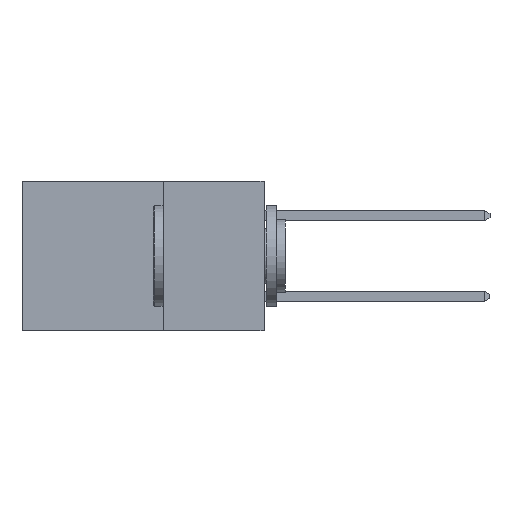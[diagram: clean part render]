
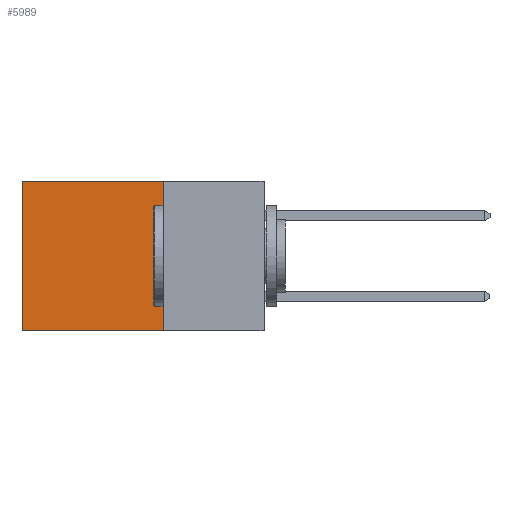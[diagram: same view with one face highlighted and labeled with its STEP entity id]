
A CAD part, left-side view. The second image highlights one B-rep face of the part: STEP entity #5989.
In plain terms, the highlighted planar face has unit normal (-1, 0, 0).
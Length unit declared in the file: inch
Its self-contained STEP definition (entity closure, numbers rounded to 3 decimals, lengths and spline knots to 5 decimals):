
#68 = LINE ( 'NONE', #2925, #7213 ) ;
#701 = ORIENTED_EDGE ( 'NONE', *, *, #2954, .F. ) ;
#1047 = CARTESIAN_POINT ( 'NONE',  ( 0.2615, 0.25, 0. ) ) ;
#1119 = ORIENTED_EDGE ( 'NONE', *, *, #8507, .F. ) ;
#2128 = ORIENTED_EDGE ( 'NONE', *, *, #4756, .T. ) ;
#2493 = VECTOR ( 'NONE', #4373, 39.37008 ) ;
#2604 = VERTEX_POINT ( 'NONE', #6181 ) ;
#2837 = PLANE ( 'NONE',  #7681 ) ;
#2925 = CARTESIAN_POINT ( 'NONE',  ( 0.2615, 0.25, -0.37 ) ) ;
#2954 = EDGE_CURVE ( 'NONE', #8616, #2604, #68, .T. ) ;
#3042 = LINE ( 'NONE', #6675, #9010 ) ;
#3496 = CARTESIAN_POINT ( 'NONE',  ( 0.2615, 0.25, -0.37 ) ) ;
#3855 = LINE ( 'NONE', #6767, #6320 ) ;
#4373 = DIRECTION ( 'NONE',  ( 0., 0., -1. ) ) ;
#4756 = EDGE_CURVE ( 'NONE', #7595, #7950, #3855, .T. ) ;
#5757 = DIRECTION ( 'NONE',  ( 0., 1., 0. ) ) ;
#5809 = LINE ( 'NONE', #9161, #2493 ) ;
#5919 = DIRECTION ( 'NONE',  ( 0., 0., -1. ) ) ;
#5989 = ADVANCED_FACE ( 'NONE', ( #7027 ), #2837, .F. ) ;
#6181 = CARTESIAN_POINT ( 'NONE',  ( 0.2615, 0.6, -0.37 ) ) ;
#6319 = DIRECTION ( 'NONE',  ( 0., 0., -1. ) ) ;
#6320 = VECTOR ( 'NONE', #7516, 39.37008 ) ;
#6550 = EDGE_CURVE ( 'NONE', #7950, #2604, #3042, .T. ) ;
#6675 = CARTESIAN_POINT ( 'NONE',  ( 0.2615, 0.6, -0.37 ) ) ;
#6767 = CARTESIAN_POINT ( 'NONE',  ( 0.2615, 0.25, 0. ) ) ;
#6798 = ORIENTED_EDGE ( 'NONE', *, *, #6550, .T. ) ;
#6910 = CARTESIAN_POINT ( 'NONE',  ( 0.2615, 0.6, 0. ) ) ;
#7027 = FACE_OUTER_BOUND ( 'NONE', #8670, .T. ) ;
#7172 = CARTESIAN_POINT ( 'NONE',  ( 0.2615, 0.25, -0.37 ) ) ;
#7213 = VECTOR ( 'NONE', #5757, 39.37008 ) ;
#7516 = DIRECTION ( 'NONE',  ( 0., 1., 0. ) ) ;
#7595 = VERTEX_POINT ( 'NONE', #1047 ) ;
#7681 = AXIS2_PLACEMENT_3D ( 'NONE', #3496, #7859, #6319 ) ;
#7859 = DIRECTION ( 'NONE',  ( 1., 0., 0. ) ) ;
#7950 = VERTEX_POINT ( 'NONE', #6910 ) ;
#8507 = EDGE_CURVE ( 'NONE', #7595, #8616, #5809, .T. ) ;
#8616 = VERTEX_POINT ( 'NONE', #7172 ) ;
#8670 = EDGE_LOOP ( 'NONE', ( #6798, #701, #1119, #2128 ) ) ;
#9010 = VECTOR ( 'NONE', #5919, 39.37008 ) ;
#9161 = CARTESIAN_POINT ( 'NONE',  ( 0.2615, 0.25, -0.37 ) ) ;
